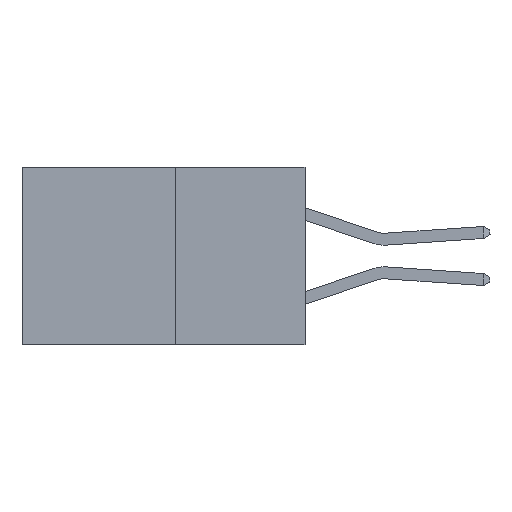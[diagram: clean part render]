
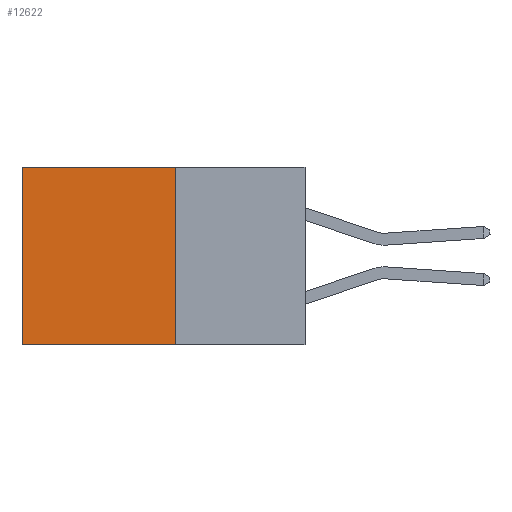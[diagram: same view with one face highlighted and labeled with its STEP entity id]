
A CAD part, left-side view. The second image highlights one B-rep face of the part: STEP entity #12622.
In plain terms, the highlighted planar face has unit normal (-1, 0, 0).
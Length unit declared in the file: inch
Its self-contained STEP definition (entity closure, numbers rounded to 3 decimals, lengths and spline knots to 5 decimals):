
#467 = ORIENTED_EDGE ( 'NONE', *, *, #7730, .F. ) ;
#1178 = DIRECTION ( 'NONE',  ( 0., 1., 0. ) ) ;
#1420 = ORIENTED_EDGE ( 'NONE', *, *, #12725, .F. ) ;
#1528 = ORIENTED_EDGE ( 'NONE', *, *, #3749, .T. ) ;
#1677 = VECTOR ( 'NONE', #1178, 39.37008 ) ;
#3069 = CARTESIAN_POINT ( 'NONE',  ( 0.277, 0.59, 0. ) ) ;
#3111 = VECTOR ( 'NONE', #8642, 39.37008 ) ;
#3749 = EDGE_CURVE ( 'NONE', #11752, #10779, #12370, .T. ) ;
#4023 = PLANE ( 'NONE',  #13836 ) ;
#4216 = CARTESIAN_POINT ( 'NONE',  ( 0.277, 0.27, -0.37 ) ) ;
#4348 = VERTEX_POINT ( 'NONE', #9981 ) ;
#4874 = EDGE_LOOP ( 'NONE', ( #12477, #1420, #467, #1528 ) ) ;
#5282 = VECTOR ( 'NONE', #19312, 39.37008 ) ;
#5582 = CARTESIAN_POINT ( 'NONE',  ( 0.277, 0.27, -0.37 ) ) ;
#6111 = LINE ( 'NONE', #4216, #1677 ) ;
#7013 = DIRECTION ( 'NONE',  ( 1., 0., 0. ) ) ;
#7036 = LINE ( 'NONE', #5582, #3111 ) ;
#7062 = FACE_OUTER_BOUND ( 'NONE', #4874, .T. ) ;
#7221 = DIRECTION ( 'NONE',  ( 0., 0., -1. ) ) ;
#7730 = EDGE_CURVE ( 'NONE', #11752, #13562, #7036, .T. ) ;
#8642 = DIRECTION ( 'NONE',  ( 0., 0., -1. ) ) ;
#9981 = CARTESIAN_POINT ( 'NONE',  ( 0.277, 0.59, -0.37 ) ) ;
#10779 = VERTEX_POINT ( 'NONE', #3069 ) ;
#11752 = VERTEX_POINT ( 'NONE', #14447 ) ;
#12370 = LINE ( 'NONE', #19113, #5282 ) ;
#12477 = ORIENTED_EDGE ( 'NONE', *, *, #17511, .T. ) ;
#12622 = ADVANCED_FACE ( 'NONE', ( #7062 ), #4023, .F. ) ;
#12725 = EDGE_CURVE ( 'NONE', #13562, #4348, #6111, .T. ) ;
#13562 = VERTEX_POINT ( 'NONE', #13949 ) ;
#13686 = VECTOR ( 'NONE', #7221, 39.37008 ) ;
#13836 = AXIS2_PLACEMENT_3D ( 'NONE', #16004, #7013, #17473 ) ;
#13949 = CARTESIAN_POINT ( 'NONE',  ( 0.277, 0.27, -0.37 ) ) ;
#14447 = CARTESIAN_POINT ( 'NONE',  ( 0.277, 0.27, 0. ) ) ;
#16004 = CARTESIAN_POINT ( 'NONE',  ( 0.277, 0.27, -0.37 ) ) ;
#16216 = CARTESIAN_POINT ( 'NONE',  ( 0.277, 0.59, -0.37 ) ) ;
#17110 = LINE ( 'NONE', #16216, #13686 ) ;
#17473 = DIRECTION ( 'NONE',  ( 0., 0., -1. ) ) ;
#17511 = EDGE_CURVE ( 'NONE', #10779, #4348, #17110, .T. ) ;
#19113 = CARTESIAN_POINT ( 'NONE',  ( 0.277, 0.27, 0. ) ) ;
#19312 = DIRECTION ( 'NONE',  ( 0., 1., 0. ) ) ;
